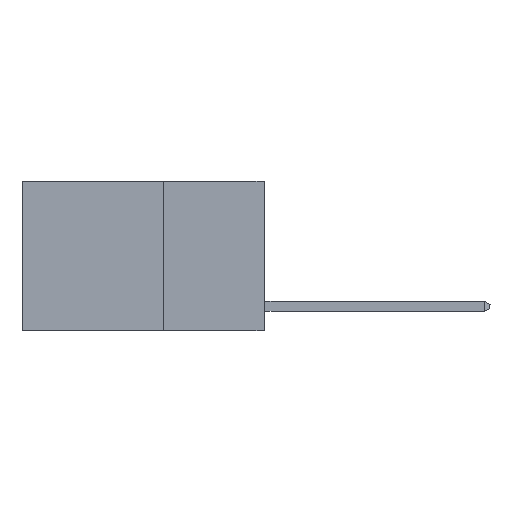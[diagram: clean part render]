
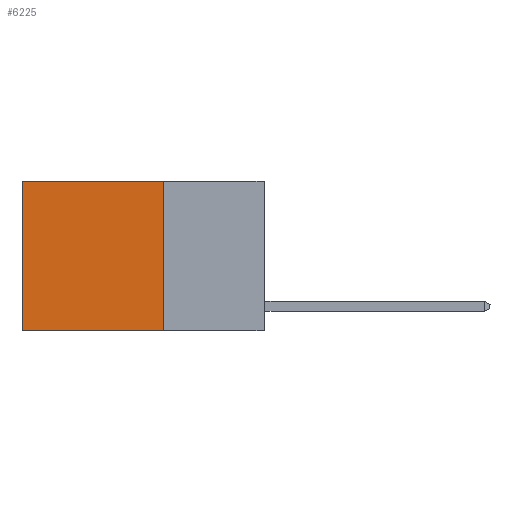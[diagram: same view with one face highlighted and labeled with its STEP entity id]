
A CAD part, left-side view. The second image highlights one B-rep face of the part: STEP entity #6225.
In plain terms, the highlighted planar face has unit normal (-1, 0, 0).
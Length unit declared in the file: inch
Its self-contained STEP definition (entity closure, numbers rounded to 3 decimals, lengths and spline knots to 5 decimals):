
#1587 = VERTEX_POINT ( 'NONE', #22803 ) ;
#2283 = ORIENTED_EDGE ( 'NONE', *, *, #23778, .T. ) ;
#2672 = CARTESIAN_POINT ( 'NONE',  ( 0.2625, 0.6, 0. ) ) ;
#3857 = DIRECTION ( 'NONE',  ( 0., 0., -1. ) ) ;
#4039 = CARTESIAN_POINT ( 'NONE',  ( 0.2625, 0.25, 0. ) ) ;
#4990 = CARTESIAN_POINT ( 'NONE',  ( 0.2625, 0.6, 0. ) ) ;
#5563 = VERTEX_POINT ( 'NONE', #6242 ) ;
#5610 = VECTOR ( 'NONE', #3857, 39.37008 ) ;
#6225 = ADVANCED_FACE ( 'NONE', ( #17136 ), #17832, .F. ) ;
#6242 = CARTESIAN_POINT ( 'NONE',  ( 0.2625, 0.25, -0.37 ) ) ;
#6410 = DIRECTION ( 'NONE',  ( 1., 0., 0. ) ) ;
#6808 = VECTOR ( 'NONE', #10007, 39.37008 ) ;
#8300 = CARTESIAN_POINT ( 'NONE',  ( 0.2625, 0.25, -0.37 ) ) ;
#8880 = CARTESIAN_POINT ( 'NONE',  ( 0.2625, 0.25, 0. ) ) ;
#10007 = DIRECTION ( 'NONE',  ( 0., 1., 0. ) ) ;
#10274 = EDGE_CURVE ( 'NONE', #26653, #1587, #28311, .T. ) ;
#11966 = EDGE_CURVE ( 'NONE', #24215, #5563, #23872, .T. ) ;
#13216 = ORIENTED_EDGE ( 'NONE', *, *, #23976, .F. ) ;
#13476 = EDGE_LOOP ( 'NONE', ( #18575, #13216, #26081, #2283 ) ) ;
#17136 = FACE_OUTER_BOUND ( 'NONE', #13476, .T. ) ;
#17332 = VECTOR ( 'NONE', #26538, 39.37008 ) ;
#17660 = CARTESIAN_POINT ( 'NONE',  ( 0.2625, 0.25, 0. ) ) ;
#17832 = PLANE ( 'NONE',  #20055 ) ;
#18575 = ORIENTED_EDGE ( 'NONE', *, *, #10274, .T. ) ;
#20055 = AXIS2_PLACEMENT_3D ( 'NONE', #4039, #6410, #22442 ) ;
#21146 = LINE ( 'NONE', #25849, #6808 ) ;
#21150 = DIRECTION ( 'NONE',  ( 0., 0., -1. ) ) ;
#22442 = DIRECTION ( 'NONE',  ( 0., 0., -1. ) ) ;
#22803 = CARTESIAN_POINT ( 'NONE',  ( 0.2625, 0.6, -0.37 ) ) ;
#22986 = VECTOR ( 'NONE', #21150, 39.37008 ) ;
#23407 = LINE ( 'NONE', #8300, #17332 ) ;
#23778 = EDGE_CURVE ( 'NONE', #24215, #26653, #21146, .T. ) ;
#23872 = LINE ( 'NONE', #17660, #5610 ) ;
#23976 = EDGE_CURVE ( 'NONE', #5563, #1587, #23407, .T. ) ;
#24215 = VERTEX_POINT ( 'NONE', #8880 ) ;
#25849 = CARTESIAN_POINT ( 'NONE',  ( 0.2625, 0.25, 0. ) ) ;
#26081 = ORIENTED_EDGE ( 'NONE', *, *, #11966, .F. ) ;
#26538 = DIRECTION ( 'NONE',  ( 0., 1., 0. ) ) ;
#26653 = VERTEX_POINT ( 'NONE', #4990 ) ;
#28311 = LINE ( 'NONE', #2672, #22986 ) ;
